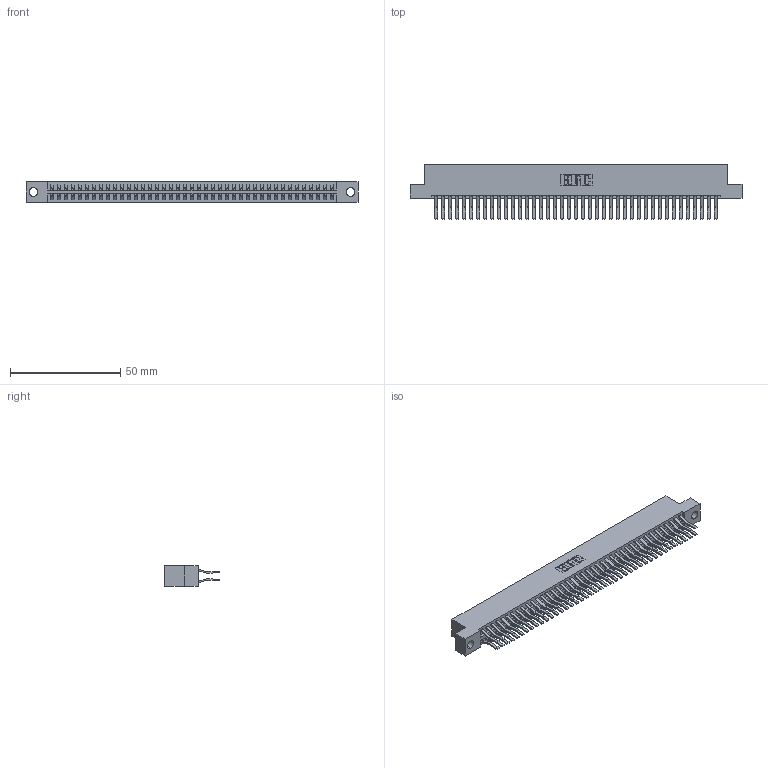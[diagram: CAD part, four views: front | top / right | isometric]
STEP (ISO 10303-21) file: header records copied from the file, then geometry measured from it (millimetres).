
FILE_DESCRIPTION (( 'STEP AP203' ), '1' );
FILE_NAME ('346-082-560-204.STEP', '2022-05-25T18:55:04', ( '' ), ( '' ), 'SwSTEP 2.0', 'SolidWorks 2020', '' );
FILE_SCHEMA (( 'CONFIG_CONTROL_DESIGN' ));
Length unit declared in the file: inch
Products named in the file (3): 345-292-001_560 Tail; 346 Part_Flush Mounting Lugs - 0.156 Dia-TH; 346-082-560-204
Assembly tree (83 placements, depth 2):
  346-082-560-204
    346 Part_Flush Mounting Lugs - 0.156 Dia-TH
    345-292-001_560 Tail  x82
Bounding box: 150.75 x 24.78 x 9.4 mm (x, y, z)
Volume: 15123.7 mm3; surface area: 22054.6 mm2
Topology: 83 solids, 83 shells, 4564 faces, 13567 edges, 8934 vertices
Faces by surface type: plane 2960, cylinder 1604
Entity records: 27399 total; most frequent: CARTESIAN_POINT 4522, ORIENTED_EDGE 4454, DIRECTION 4039, EDGE_CURVE 2227, VECTOR 1927, LINE 1927, VERTEX_POINT 1482, AXIS2_PLACEMENT_3D 1056
